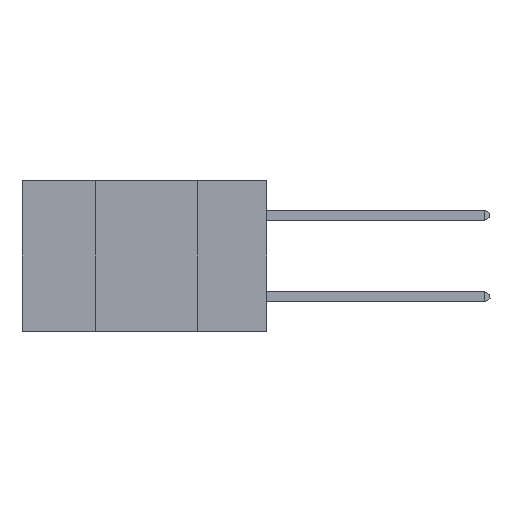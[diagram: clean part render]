
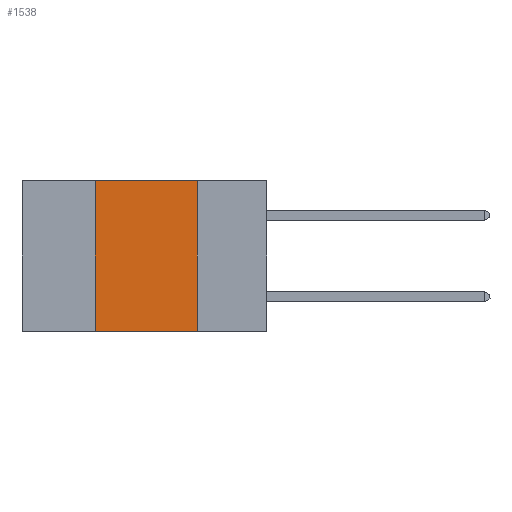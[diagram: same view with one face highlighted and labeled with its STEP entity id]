
A CAD part, left-side view. The second image highlights one B-rep face of the part: STEP entity #1538.
In plain terms, the highlighted planar face has unit normal (-1, 0, 0).
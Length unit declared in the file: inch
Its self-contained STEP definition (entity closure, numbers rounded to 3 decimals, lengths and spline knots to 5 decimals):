
#1407 = CARTESIAN_POINT ( 'NONE',  ( 0., 0.6, -0.37 ) ) ;
#1538 = ADVANCED_FACE ( 'NONE', ( #10019 ), #20313, .F. ) ;
#2489 = CARTESIAN_POINT ( 'NONE',  ( 0., 0.42, 0. ) ) ;
#3764 = EDGE_CURVE ( 'NONE', #5325, #4244, #9763, .T. ) ;
#4244 = VERTEX_POINT ( 'NONE', #16955 ) ;
#4595 = VERTEX_POINT ( 'NONE', #22393 ) ;
#4778 = EDGE_CURVE ( 'NONE', #5901, #5325, #14573, .T. ) ;
#4911 = AXIS2_PLACEMENT_3D ( 'NONE', #22291, #9219, #7373 ) ;
#5203 = DIRECTION ( 'NONE',  ( 0., 0., -1. ) ) ;
#5325 = VERTEX_POINT ( 'NONE', #5838 ) ;
#5838 = CARTESIAN_POINT ( 'NONE',  ( 0., 0.17, 0. ) ) ;
#5901 = VERTEX_POINT ( 'NONE', #2489 ) ;
#7022 = ORIENTED_EDGE ( 'NONE', *, *, #11111, .T. ) ;
#7373 = DIRECTION ( 'NONE',  ( 0., 0., -1. ) ) ;
#7463 = VECTOR ( 'NONE', #22030, 39.37008 ) ;
#7506 = EDGE_CURVE ( 'NONE', #4595, #5901, #21502, .T. ) ;
#8032 = DIRECTION ( 'NONE',  ( 0., -1., 0. ) ) ;
#8106 = LINE ( 'NONE', #1407, #22462 ) ;
#8557 = VECTOR ( 'NONE', #5203, 39.37008 ) ;
#9219 = DIRECTION ( 'NONE',  ( 1., 0., 0. ) ) ;
#9763 = LINE ( 'NONE', #16846, #8557 ) ;
#10019 = FACE_OUTER_BOUND ( 'NONE', #21420, .T. ) ;
#10597 = VECTOR ( 'NONE', #8032, 39.37008 ) ;
#11111 = EDGE_CURVE ( 'NONE', #4595, #4244, #8106, .T. ) ;
#13480 = ORIENTED_EDGE ( 'NONE', *, *, #4778, .F. ) ;
#14573 = LINE ( 'NONE', #20651, #10597 ) ;
#14892 = DIRECTION ( 'NONE',  ( 0., -1., 0. ) ) ;
#16384 = CARTESIAN_POINT ( 'NONE',  ( 0., 0.42, 0. ) ) ;
#16846 = CARTESIAN_POINT ( 'NONE',  ( 0., 0.17, 0. ) ) ;
#16955 = CARTESIAN_POINT ( 'NONE',  ( 0., 0.17, -0.37 ) ) ;
#20313 = PLANE ( 'NONE',  #4911 ) ;
#20651 = CARTESIAN_POINT ( 'NONE',  ( 0., 0.6, 0. ) ) ;
#20937 = ORIENTED_EDGE ( 'NONE', *, *, #3764, .F. ) ;
#21420 = EDGE_LOOP ( 'NONE', ( #20937, #13480, #24797, #7022 ) ) ;
#21502 = LINE ( 'NONE', #16384, #7463 ) ;
#22030 = DIRECTION ( 'NONE',  ( 0., 0., 1. ) ) ;
#22291 = CARTESIAN_POINT ( 'NONE',  ( 0., 0.6, 0. ) ) ;
#22393 = CARTESIAN_POINT ( 'NONE',  ( 0., 0.42, -0.37 ) ) ;
#22462 = VECTOR ( 'NONE', #14892, 39.37008 ) ;
#24797 = ORIENTED_EDGE ( 'NONE', *, *, #7506, .F. ) ;
